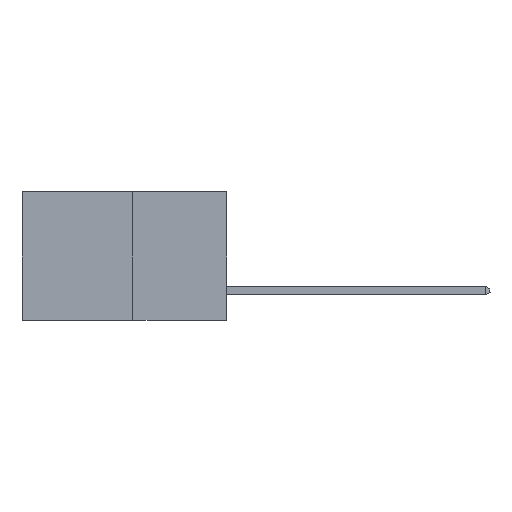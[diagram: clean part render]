
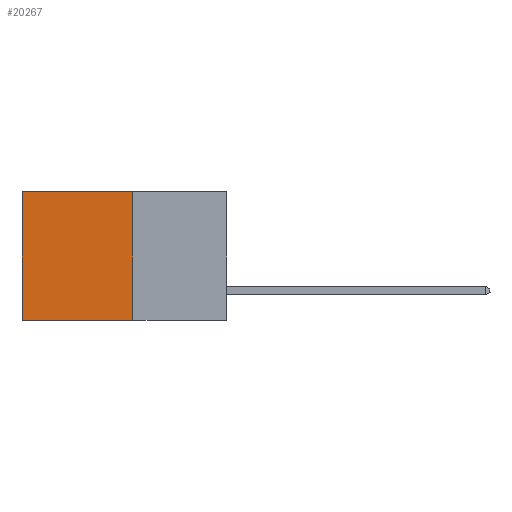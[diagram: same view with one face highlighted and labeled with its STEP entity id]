
A CAD part, left-side view. The second image highlights one B-rep face of the part: STEP entity #20267.
In plain terms, the highlighted planar face has unit normal (-1, 0, 0).
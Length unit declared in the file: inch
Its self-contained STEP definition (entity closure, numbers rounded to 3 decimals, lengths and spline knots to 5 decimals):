
#761 = VECTOR ( 'NONE', #11981, 39.37008 ) ;
#995 = VECTOR ( 'NONE', #10691, 39.37008 ) ;
#1684 = CARTESIAN_POINT ( 'NONE',  ( 0.277, 0.27, -0.37 ) ) ;
#1712 = CARTESIAN_POINT ( 'NONE',  ( 0.277, 0.27, 0. ) ) ;
#2631 = EDGE_LOOP ( 'NONE', ( #20618, #14702, #6646, #17916 ) ) ;
#2760 = CARTESIAN_POINT ( 'NONE',  ( 0.277, 0.27, -0.37 ) ) ;
#3614 = CARTESIAN_POINT ( 'NONE',  ( 0.277, 0.27, 0. ) ) ;
#5326 = EDGE_CURVE ( 'NONE', #8055, #19072, #18586, .T. ) ;
#5874 = AXIS2_PLACEMENT_3D ( 'NONE', #2760, #6295, #18271 ) ;
#6259 = CARTESIAN_POINT ( 'NONE',  ( 0.277, 0.27, -0.37 ) ) ;
#6295 = DIRECTION ( 'NONE',  ( 1., 0., 0. ) ) ;
#6413 = EDGE_CURVE ( 'NONE', #18797, #6578, #18795, .T. ) ;
#6465 = FACE_OUTER_BOUND ( 'NONE', #2631, .T. ) ;
#6578 = VERTEX_POINT ( 'NONE', #6259 ) ;
#6646 = ORIENTED_EDGE ( 'NONE', *, *, #6413, .F. ) ;
#8055 = VERTEX_POINT ( 'NONE', #20789 ) ;
#10459 = LINE ( 'NONE', #1712, #20009 ) ;
#10691 = DIRECTION ( 'NONE',  ( 0., 0., -1. ) ) ;
#10898 = CARTESIAN_POINT ( 'NONE',  ( 0.277, 0.59, -0.37 ) ) ;
#11981 = DIRECTION ( 'NONE',  ( 0., 0., -1. ) ) ;
#13837 = DIRECTION ( 'NONE',  ( 0., 1., 0. ) ) ;
#14622 = EDGE_CURVE ( 'NONE', #18797, #8055, #10459, .T. ) ;
#14702 = ORIENTED_EDGE ( 'NONE', *, *, #21266, .F. ) ;
#16134 = VECTOR ( 'NONE', #19168, 39.37008 ) ;
#16602 = PLANE ( 'NONE',  #5874 ) ;
#17521 = CARTESIAN_POINT ( 'NONE',  ( 0.277, 0.27, -0.37 ) ) ;
#17916 = ORIENTED_EDGE ( 'NONE', *, *, #14622, .T. ) ;
#18271 = DIRECTION ( 'NONE',  ( 0., 0., -1. ) ) ;
#18530 = CARTESIAN_POINT ( 'NONE',  ( 0.277, 0.59, -0.37 ) ) ;
#18586 = LINE ( 'NONE', #10898, #761 ) ;
#18795 = LINE ( 'NONE', #1684, #995 ) ;
#18797 = VERTEX_POINT ( 'NONE', #3614 ) ;
#19072 = VERTEX_POINT ( 'NONE', #18530 ) ;
#19168 = DIRECTION ( 'NONE',  ( 0., 1., 0. ) ) ;
#20009 = VECTOR ( 'NONE', #13837, 39.37008 ) ;
#20044 = LINE ( 'NONE', #17521, #16134 ) ;
#20267 = ADVANCED_FACE ( 'NONE', ( #6465 ), #16602, .F. ) ;
#20618 = ORIENTED_EDGE ( 'NONE', *, *, #5326, .T. ) ;
#20789 = CARTESIAN_POINT ( 'NONE',  ( 0.277, 0.59, 0. ) ) ;
#21266 = EDGE_CURVE ( 'NONE', #6578, #19072, #20044, .T. ) ;
